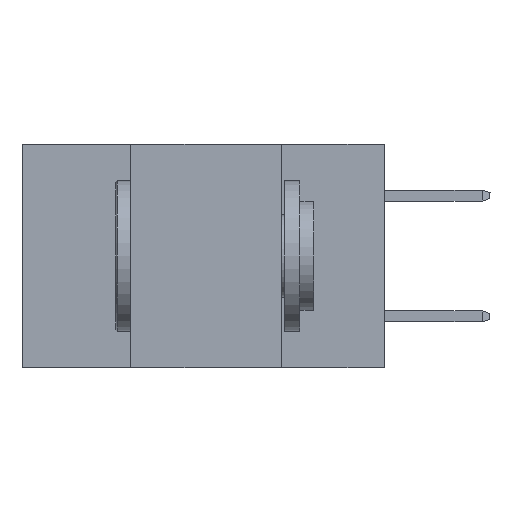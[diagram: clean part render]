
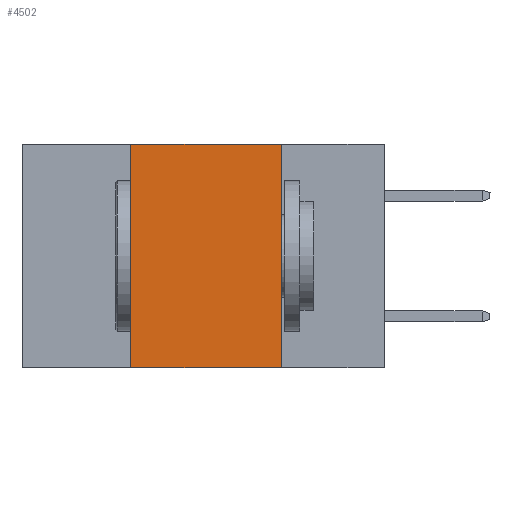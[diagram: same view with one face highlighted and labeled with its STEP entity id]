
A CAD part, left-side view. The second image highlights one B-rep face of the part: STEP entity #4502.
In plain terms, the highlighted planar face has unit normal (-1, 0, 0).
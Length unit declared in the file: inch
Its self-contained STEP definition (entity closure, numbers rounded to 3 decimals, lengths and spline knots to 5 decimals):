
#337 = VERTEX_POINT ( 'NONE', #12317 ) ;
#350 = VERTEX_POINT ( 'NONE', #7584 ) ;
#833 = VERTEX_POINT ( 'NONE', #4109 ) ;
#1178 = DIRECTION ( 'NONE',  ( 0., -1., 0. ) ) ;
#1448 = VECTOR ( 'NONE', #15946, 39.37008 ) ;
#2668 = ORIENTED_EDGE ( 'NONE', *, *, #4163, .T. ) ;
#3885 = EDGE_CURVE ( 'NONE', #833, #337, #19201, .T. ) ;
#4039 = CARTESIAN_POINT ( 'NONE',  ( 0., 0.6, 0. ) ) ;
#4109 = CARTESIAN_POINT ( 'NONE',  ( 0., 0.42, 0. ) ) ;
#4163 = EDGE_CURVE ( 'NONE', #350, #5903, #12712, .T. ) ;
#4464 = CARTESIAN_POINT ( 'NONE',  ( 0., 0.6, 0. ) ) ;
#4502 = ADVANCED_FACE ( 'NONE', ( #4789 ), #15112, .F. ) ;
#4582 = EDGE_LOOP ( 'NONE', ( #16696, #5909, #18834, #2668 ) ) ;
#4789 = FACE_OUTER_BOUND ( 'NONE', #4582, .T. ) ;
#5740 = VECTOR ( 'NONE', #16488, 39.37008 ) ;
#5903 = VERTEX_POINT ( 'NONE', #15044 ) ;
#5909 = ORIENTED_EDGE ( 'NONE', *, *, #3885, .F. ) ;
#6260 = CARTESIAN_POINT ( 'NONE',  ( 0., 0.6, -0.37 ) ) ;
#7557 = VECTOR ( 'NONE', #16931, 39.37008 ) ;
#7579 = DIRECTION ( 'NONE',  ( 1., 0., 0. ) ) ;
#7584 = CARTESIAN_POINT ( 'NONE',  ( 0., 0.42, -0.37 ) ) ;
#7888 = CARTESIAN_POINT ( 'NONE',  ( 0., 0.17, 0. ) ) ;
#8058 = AXIS2_PLACEMENT_3D ( 'NONE', #4464, #7579, #10455 ) ;
#9758 = EDGE_CURVE ( 'NONE', #337, #5903, #11508, .T. ) ;
#10455 = DIRECTION ( 'NONE',  ( 0., 0., -1. ) ) ;
#11374 = EDGE_CURVE ( 'NONE', #350, #833, #17431, .T. ) ;
#11397 = CARTESIAN_POINT ( 'NONE',  ( 0., 0.42, 0. ) ) ;
#11508 = LINE ( 'NONE', #7888, #7557 ) ;
#12317 = CARTESIAN_POINT ( 'NONE',  ( 0., 0.17, 0. ) ) ;
#12712 = LINE ( 'NONE', #6260, #5740 ) ;
#15044 = CARTESIAN_POINT ( 'NONE',  ( 0., 0.17, -0.37 ) ) ;
#15112 = PLANE ( 'NONE',  #8058 ) ;
#15946 = DIRECTION ( 'NONE',  ( 0., 0., 1. ) ) ;
#16488 = DIRECTION ( 'NONE',  ( 0., -1., 0. ) ) ;
#16653 = VECTOR ( 'NONE', #1178, 39.37008 ) ;
#16696 = ORIENTED_EDGE ( 'NONE', *, *, #9758, .F. ) ;
#16931 = DIRECTION ( 'NONE',  ( 0., 0., -1. ) ) ;
#17431 = LINE ( 'NONE', #11397, #1448 ) ;
#18834 = ORIENTED_EDGE ( 'NONE', *, *, #11374, .F. ) ;
#19201 = LINE ( 'NONE', #4039, #16653 ) ;
